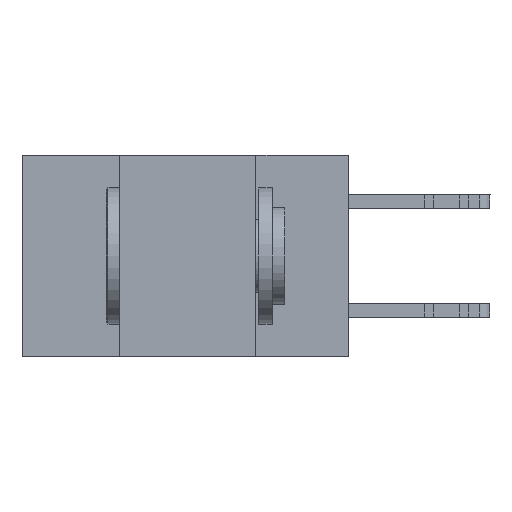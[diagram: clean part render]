
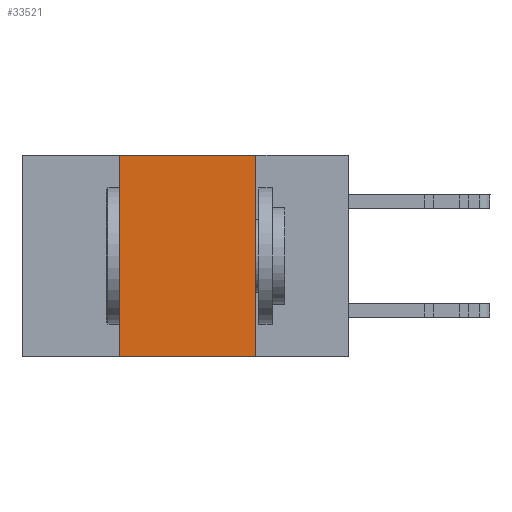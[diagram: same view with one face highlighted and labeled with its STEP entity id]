
A CAD part, left-side view. The second image highlights one B-rep face of the part: STEP entity #33521.
In plain terms, the highlighted planar face has unit normal (-1, 0, 0).
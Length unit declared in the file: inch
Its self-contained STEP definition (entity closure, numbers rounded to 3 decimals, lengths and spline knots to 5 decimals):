
#58 = DIRECTION ( 'NONE',  ( 0., 0., -1. ) ) ;
#730 = AXIS2_PLACEMENT_3D ( 'NONE', #5041, #23933, #58 ) ;
#737 = EDGE_CURVE ( 'NONE', #6942, #1390, #7455, .T. ) ;
#1390 = VERTEX_POINT ( 'NONE', #7737 ) ;
#1931 = CARTESIAN_POINT ( 'NONE',  ( 0., 0.6, -0.37 ) ) ;
#2020 = EDGE_LOOP ( 'NONE', ( #4092, #6959, #2861, #26068 ) ) ;
#2176 = VECTOR ( 'NONE', #4844, 39.37008 ) ;
#2240 = DIRECTION ( 'NONE',  ( 0., 0., 1. ) ) ;
#2317 = VERTEX_POINT ( 'NONE', #8982 ) ;
#2861 = ORIENTED_EDGE ( 'NONE', *, *, #24143, .F. ) ;
#4092 = ORIENTED_EDGE ( 'NONE', *, *, #10239, .F. ) ;
#4844 = DIRECTION ( 'NONE',  ( 0., -1., 0. ) ) ;
#5041 = CARTESIAN_POINT ( 'NONE',  ( 0., 0.6, 0. ) ) ;
#6127 = VECTOR ( 'NONE', #2240, 39.37008 ) ;
#6942 = VERTEX_POINT ( 'NONE', #10416 ) ;
#6959 = ORIENTED_EDGE ( 'NONE', *, *, #24921, .F. ) ;
#7455 = LINE ( 'NONE', #1931, #2176 ) ;
#7639 = FACE_OUTER_BOUND ( 'NONE', #2020, .T. ) ;
#7737 = CARTESIAN_POINT ( 'NONE',  ( 0., 0.17, -0.37 ) ) ;
#7794 = VECTOR ( 'NONE', #23094, 39.37008 ) ;
#8982 = CARTESIAN_POINT ( 'NONE',  ( 0., 0.42, 0. ) ) ;
#10239 = EDGE_CURVE ( 'NONE', #21352, #1390, #13739, .T. ) ;
#10378 = CARTESIAN_POINT ( 'NONE',  ( 0., 0.17, 0. ) ) ;
#10416 = CARTESIAN_POINT ( 'NONE',  ( 0., 0.42, -0.37 ) ) ;
#13739 = LINE ( 'NONE', #21660, #29624 ) ;
#15303 = LINE ( 'NONE', #23217, #6127 ) ;
#17424 = CARTESIAN_POINT ( 'NONE',  ( 0., 0.6, 0. ) ) ;
#21213 = PLANE ( 'NONE',  #730 ) ;
#21352 = VERTEX_POINT ( 'NONE', #10378 ) ;
#21660 = CARTESIAN_POINT ( 'NONE',  ( 0., 0.17, 0. ) ) ;
#22762 = LINE ( 'NONE', #17424, #7794 ) ;
#23094 = DIRECTION ( 'NONE',  ( 0., -1., 0. ) ) ;
#23217 = CARTESIAN_POINT ( 'NONE',  ( 0., 0.42, 0. ) ) ;
#23933 = DIRECTION ( 'NONE',  ( 1., 0., 0. ) ) ;
#24143 = EDGE_CURVE ( 'NONE', #6942, #2317, #15303, .T. ) ;
#24921 = EDGE_CURVE ( 'NONE', #2317, #21352, #22762, .T. ) ;
#26068 = ORIENTED_EDGE ( 'NONE', *, *, #737, .T. ) ;
#29624 = VECTOR ( 'NONE', #29897, 39.37008 ) ;
#29897 = DIRECTION ( 'NONE',  ( 0., 0., -1. ) ) ;
#33521 = ADVANCED_FACE ( 'NONE', ( #7639 ), #21213, .F. ) ;
